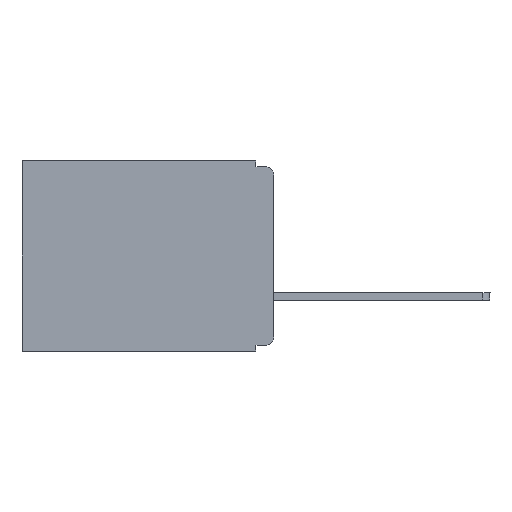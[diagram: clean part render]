
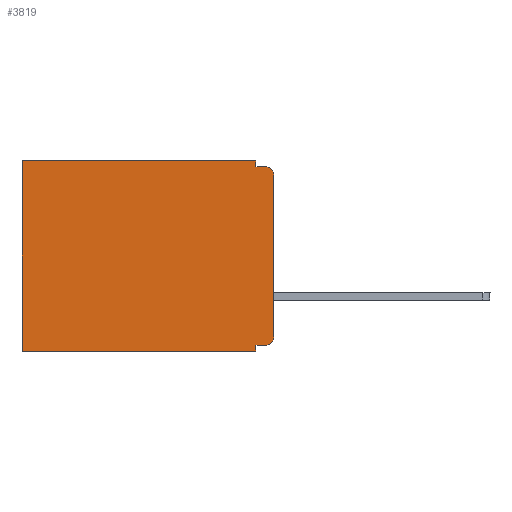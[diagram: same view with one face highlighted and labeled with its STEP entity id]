
A CAD part, left-side view. The second image highlights one B-rep face of the part: STEP entity #3819.
In plain terms, the highlighted planar face has unit normal (-1, 0, 0).
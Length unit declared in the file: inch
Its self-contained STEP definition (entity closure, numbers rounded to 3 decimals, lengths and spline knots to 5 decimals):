
#342 = ORIENTED_EDGE ( 'NONE', *, *, #14430, .F. ) ;
#651 = VECTOR ( 'NONE', #12246, 39.37008 ) ;
#910 = AXIS2_PLACEMENT_3D ( 'NONE', #2370, #7980, #2326 ) ;
#939 = DIRECTION ( 'NONE',  ( 0., 0., -1. ) ) ;
#1003 = VERTEX_POINT ( 'NONE', #11218 ) ;
#1018 = ORIENTED_EDGE ( 'NONE', *, *, #3068, .F. ) ;
#1251 = VERTEX_POINT ( 'NONE', #3751 ) ;
#1340 = DIRECTION ( 'NONE',  ( 0., 0., -1. ) ) ;
#1536 = VERTEX_POINT ( 'NONE', #1907 ) ;
#1633 = CIRCLE ( 'NONE', #910, 0.015 ) ;
#1837 = FACE_OUTER_BOUND ( 'NONE', #7148, .T. ) ;
#1907 = CARTESIAN_POINT ( 'NONE',  ( 0.3, 0., -0.305 ) ) ;
#2102 = LINE ( 'NONE', #3209, #651 ) ;
#2216 = DIRECTION ( 'NONE',  ( 0., 0., -1. ) ) ;
#2326 = DIRECTION ( 'NONE',  ( 0., 0., -1. ) ) ;
#2370 = CARTESIAN_POINT ( 'NONE',  ( 0.3, 0.015, -0.025 ) ) ;
#2767 = CARTESIAN_POINT ( 'NONE',  ( 0.3, 0., -0.33 ) ) ;
#2855 = VERTEX_POINT ( 'NONE', #13038 ) ;
#3068 = EDGE_CURVE ( 'NONE', #5912, #1003, #10390, .T. ) ;
#3199 = VERTEX_POINT ( 'NONE', #12559 ) ;
#3209 = CARTESIAN_POINT ( 'NONE',  ( 0.3, 0., -0.32 ) ) ;
#3436 = PLANE ( 'NONE',  #7447 ) ;
#3751 = CARTESIAN_POINT ( 'NONE',  ( 0.3, 0.015, -0.01 ) ) ;
#3817 = DIRECTION ( 'NONE',  ( 0., 0., -1. ) ) ;
#3819 = ADVANCED_FACE ( 'NONE', ( #1837 ), #3436, .F. ) ;
#4327 = CIRCLE ( 'NONE', #12175, 0.015 ) ;
#4473 = DIRECTION ( 'NONE',  ( 0., 0., -1. ) ) ;
#4761 = DIRECTION ( 'NONE',  ( 1., 0., 0. ) ) ;
#5265 = CARTESIAN_POINT ( 'NONE',  ( 0.3, 0., -0.025 ) ) ;
#5701 = CARTESIAN_POINT ( 'NONE',  ( 0.3, 0.015, -0.305 ) ) ;
#5746 = ORIENTED_EDGE ( 'NONE', *, *, #10445, .F. ) ;
#5912 = VERTEX_POINT ( 'NONE', #8761 ) ;
#6110 = VECTOR ( 'NONE', #12335, 39.37008 ) ;
#6161 = CARTESIAN_POINT ( 'NONE',  ( 0.3, 0., 0. ) ) ;
#6465 = ORIENTED_EDGE ( 'NONE', *, *, #10819, .T. ) ;
#6565 = VECTOR ( 'NONE', #3817, 39.37008 ) ;
#6578 = LINE ( 'NONE', #2767, #14622 ) ;
#6694 = CARTESIAN_POINT ( 'NONE',  ( 0.3, 0.031, -0.33 ) ) ;
#6727 = LINE ( 'NONE', #6694, #13870 ) ;
#6782 = VERTEX_POINT ( 'NONE', #7318 ) ;
#6790 = VECTOR ( 'NONE', #9949, 39.37008 ) ;
#6823 = DIRECTION ( 'NONE',  ( -1., 0., 0. ) ) ;
#7142 = ORIENTED_EDGE ( 'NONE', *, *, #9299, .T. ) ;
#7148 = EDGE_LOOP ( 'NONE', ( #11325, #9177, #342, #1018, #8881, #6465, #11287, #5746, #12839, #7142 ) ) ;
#7289 = EDGE_CURVE ( 'NONE', #3199, #11440, #2102, .T. ) ;
#7318 = CARTESIAN_POINT ( 'NONE',  ( 0.3, 0.031, -0.33 ) ) ;
#7447 = AXIS2_PLACEMENT_3D ( 'NONE', #11554, #4761, #1340 ) ;
#7645 = CARTESIAN_POINT ( 'NONE',  ( 0.3, 0., -0.01 ) ) ;
#7980 = DIRECTION ( 'NONE',  ( -1., 0., 0. ) ) ;
#8710 = CARTESIAN_POINT ( 'NONE',  ( 0.3, 0.437, -0.33 ) ) ;
#8761 = CARTESIAN_POINT ( 'NONE',  ( 0.3, 0.031, 0. ) ) ;
#8881 = ORIENTED_EDGE ( 'NONE', *, *, #11233, .T. ) ;
#9054 = EDGE_CURVE ( 'NONE', #6782, #11131, #6578, .T. ) ;
#9149 = LINE ( 'NONE', #7645, #6790 ) ;
#9177 = ORIENTED_EDGE ( 'NONE', *, *, #11038, .T. ) ;
#9242 = VECTOR ( 'NONE', #10708, 39.37008 ) ;
#9299 = EDGE_CURVE ( 'NONE', #3199, #1536, #4327, .T. ) ;
#9474 = CARTESIAN_POINT ( 'NONE',  ( 0.3, 0.437, -0.33 ) ) ;
#9543 = EDGE_CURVE ( 'NONE', #10027, #1536, #11934, .T. ) ;
#9949 = DIRECTION ( 'NONE',  ( 0., -1., 0. ) ) ;
#10027 = VERTEX_POINT ( 'NONE', #5265 ) ;
#10390 = LINE ( 'NONE', #12200, #6110 ) ;
#10445 = EDGE_CURVE ( 'NONE', #11440, #6782, #6727, .T. ) ;
#10580 = CARTESIAN_POINT ( 'NONE',  ( 0.3, 0., -0.33 ) ) ;
#10708 = DIRECTION ( 'NONE',  ( 0., 1., 0. ) ) ;
#10819 = EDGE_CURVE ( 'NONE', #2855, #11131, #13333, .T. ) ;
#10874 = DIRECTION ( 'NONE',  ( 0., 1., 0. ) ) ;
#11038 = EDGE_CURVE ( 'NONE', #10027, #1251, #1633, .T. ) ;
#11131 = VERTEX_POINT ( 'NONE', #9474 ) ;
#11218 = CARTESIAN_POINT ( 'NONE',  ( 0.3, 0.031, -0.01 ) ) ;
#11233 = EDGE_CURVE ( 'NONE', #5912, #2855, #14387, .T. ) ;
#11287 = ORIENTED_EDGE ( 'NONE', *, *, #9054, .F. ) ;
#11325 = ORIENTED_EDGE ( 'NONE', *, *, #9543, .F. ) ;
#11440 = VERTEX_POINT ( 'NONE', #12134 ) ;
#11554 = CARTESIAN_POINT ( 'NONE',  ( 0.3, 0., -0.33 ) ) ;
#11934 = LINE ( 'NONE', #10580, #6565 ) ;
#12134 = CARTESIAN_POINT ( 'NONE',  ( 0.3, 0.031, -0.32 ) ) ;
#12175 = AXIS2_PLACEMENT_3D ( 'NONE', #5701, #6823, #4473 ) ;
#12200 = CARTESIAN_POINT ( 'NONE',  ( 0.3, 0.031, 0. ) ) ;
#12246 = DIRECTION ( 'NONE',  ( 0., 1., 0. ) ) ;
#12264 = VECTOR ( 'NONE', #939, 39.37008 ) ;
#12335 = DIRECTION ( 'NONE',  ( 0., 0., -1. ) ) ;
#12559 = CARTESIAN_POINT ( 'NONE',  ( 0.3, 0.015, -0.32 ) ) ;
#12839 = ORIENTED_EDGE ( 'NONE', *, *, #7289, .F. ) ;
#13038 = CARTESIAN_POINT ( 'NONE',  ( 0.3, 0.437, 0. ) ) ;
#13333 = LINE ( 'NONE', #8710, #12264 ) ;
#13870 = VECTOR ( 'NONE', #2216, 39.37008 ) ;
#14387 = LINE ( 'NONE', #6161, #9242 ) ;
#14430 = EDGE_CURVE ( 'NONE', #1003, #1251, #9149, .T. ) ;
#14622 = VECTOR ( 'NONE', #10874, 39.37008 ) ;
